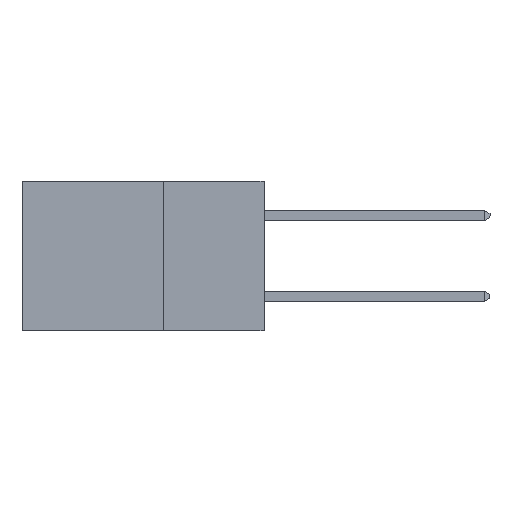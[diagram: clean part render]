
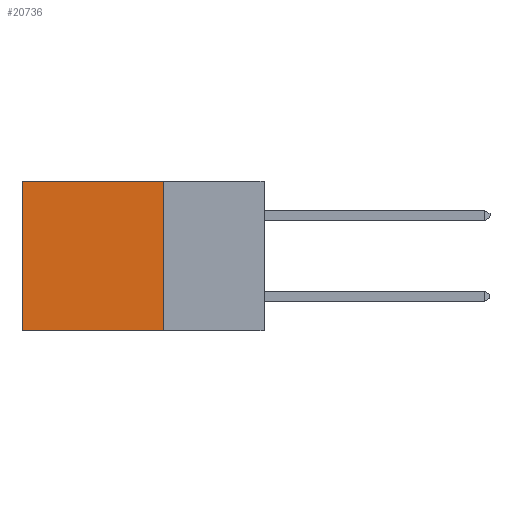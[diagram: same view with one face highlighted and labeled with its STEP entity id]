
A CAD part, left-side view. The second image highlights one B-rep face of the part: STEP entity #20736.
In plain terms, the highlighted planar face has unit normal (-1, 0, 0).
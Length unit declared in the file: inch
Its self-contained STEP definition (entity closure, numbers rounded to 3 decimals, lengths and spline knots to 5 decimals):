
#1105 = CARTESIAN_POINT ( 'NONE',  ( 0.298, 0.25, 0. ) ) ;
#1329 = VECTOR ( 'NONE', #20860, 39.37008 ) ;
#1694 = VECTOR ( 'NONE', #11075, 39.37008 ) ;
#2377 = LINE ( 'NONE', #8922, #1694 ) ;
#2989 = FACE_OUTER_BOUND ( 'NONE', #17727, .T. ) ;
#3279 = DIRECTION ( 'NONE',  ( 0., 0., -1. ) ) ;
#5816 = VERTEX_POINT ( 'NONE', #11015 ) ;
#6688 = AXIS2_PLACEMENT_3D ( 'NONE', #1105, #16065, #3279 ) ;
#8221 = CARTESIAN_POINT ( 'NONE',  ( 0.298, 0.25, -0.37 ) ) ;
#8922 = CARTESIAN_POINT ( 'NONE',  ( 0.298, 0.25, 0. ) ) ;
#10292 = CARTESIAN_POINT ( 'NONE',  ( 0.298, 0.6, 0. ) ) ;
#10608 = CARTESIAN_POINT ( 'NONE',  ( 0.298, 0.25, 0. ) ) ;
#11015 = CARTESIAN_POINT ( 'NONE',  ( 0.298, 0.6, -0.37 ) ) ;
#11075 = DIRECTION ( 'NONE',  ( 0., 1., 0. ) ) ;
#13888 = EDGE_CURVE ( 'NONE', #18743, #5816, #17709, .T. ) ;
#15378 = EDGE_CURVE ( 'NONE', #24416, #5816, #27374, .T. ) ;
#15585 = ORIENTED_EDGE ( 'NONE', *, *, #19736, .F. ) ;
#15593 = VERTEX_POINT ( 'NONE', #21433 ) ;
#16065 = DIRECTION ( 'NONE',  ( 1., 0., 0. ) ) ;
#16080 = CARTESIAN_POINT ( 'NONE',  ( 0.298, 0.25, -0.37 ) ) ;
#16277 = VECTOR ( 'NONE', #27036, 39.37008 ) ;
#17709 = LINE ( 'NONE', #8221, #1329 ) ;
#17727 = EDGE_LOOP ( 'NONE', ( #27111, #25417, #15585, #18512 ) ) ;
#17729 = VECTOR ( 'NONE', #21276, 39.37008 ) ;
#18512 = ORIENTED_EDGE ( 'NONE', *, *, #23674, .T. ) ;
#18743 = VERTEX_POINT ( 'NONE', #16080 ) ;
#19736 = EDGE_CURVE ( 'NONE', #15593, #18743, #24626, .T. ) ;
#20736 = ADVANCED_FACE ( 'NONE', ( #2989 ), #24432, .F. ) ;
#20860 = DIRECTION ( 'NONE',  ( 0., 1., 0. ) ) ;
#21276 = DIRECTION ( 'NONE',  ( 0., 0., -1. ) ) ;
#21433 = CARTESIAN_POINT ( 'NONE',  ( 0.298, 0.25, 0. ) ) ;
#22361 = CARTESIAN_POINT ( 'NONE',  ( 0.298, 0.6, 0. ) ) ;
#23674 = EDGE_CURVE ( 'NONE', #15593, #24416, #2377, .T. ) ;
#24416 = VERTEX_POINT ( 'NONE', #22361 ) ;
#24432 = PLANE ( 'NONE',  #6688 ) ;
#24626 = LINE ( 'NONE', #10608, #17729 ) ;
#25417 = ORIENTED_EDGE ( 'NONE', *, *, #13888, .F. ) ;
#27036 = DIRECTION ( 'NONE',  ( 0., 0., -1. ) ) ;
#27111 = ORIENTED_EDGE ( 'NONE', *, *, #15378, .T. ) ;
#27374 = LINE ( 'NONE', #10292, #16277 ) ;
